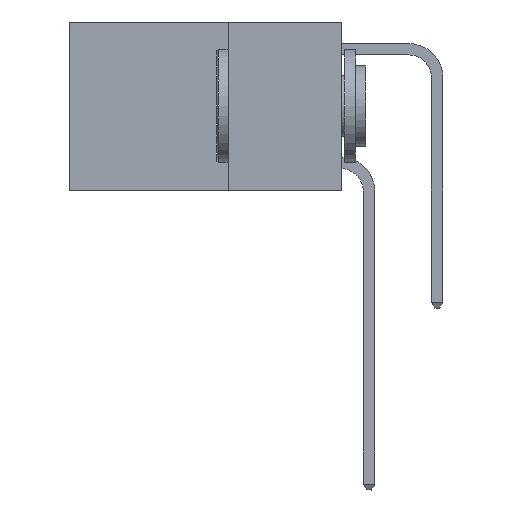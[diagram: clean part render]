
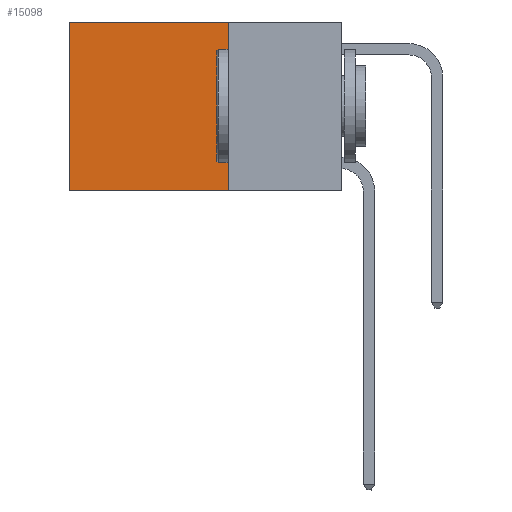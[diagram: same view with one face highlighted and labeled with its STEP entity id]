
A CAD part, left-side view. The second image highlights one B-rep face of the part: STEP entity #15098.
In plain terms, the highlighted planar face has unit normal (-1, 0, 0).
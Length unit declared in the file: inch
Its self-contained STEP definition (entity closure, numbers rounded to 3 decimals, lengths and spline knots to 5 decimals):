
#177 = VERTEX_POINT ( 'NONE', #13734 ) ;
#1425 = EDGE_LOOP ( 'NONE', ( #12288, #14603, #14387, #11942 ) ) ;
#2439 = LINE ( 'NONE', #4315, #9873 ) ;
#3101 = DIRECTION ( 'NONE',  ( 0., 0., -1. ) ) ;
#3390 = FACE_OUTER_BOUND ( 'NONE', #1425, .T. ) ;
#4002 = LINE ( 'NONE', #7908, #15254 ) ;
#4315 = CARTESIAN_POINT ( 'NONE',  ( 0.2625, 0.25, -0.37 ) ) ;
#5177 = DIRECTION ( 'NONE',  ( 0., 1., 0. ) ) ;
#5392 = CARTESIAN_POINT ( 'NONE',  ( 0.2625, 0.25, -0.37 ) ) ;
#5939 = VERTEX_POINT ( 'NONE', #7445 ) ;
#6036 = CARTESIAN_POINT ( 'NONE',  ( 0.2625, 0.25, 0. ) ) ;
#6421 = DIRECTION ( 'NONE',  ( 0., 0., -1. ) ) ;
#7288 = DIRECTION ( 'NONE',  ( 0., 1., 0. ) ) ;
#7445 = CARTESIAN_POINT ( 'NONE',  ( 0.2625, 0.6, 0. ) ) ;
#7856 = CARTESIAN_POINT ( 'NONE',  ( 0.2625, 0.6, -0.37 ) ) ;
#7908 = CARTESIAN_POINT ( 'NONE',  ( 0.2625, 0.25, 0. ) ) ;
#8926 = LINE ( 'NONE', #17455, #9383 ) ;
#9383 = VECTOR ( 'NONE', #18900, 39.37008 ) ;
#9873 = VECTOR ( 'NONE', #7288, 39.37008 ) ;
#10489 = VERTEX_POINT ( 'NONE', #7856 ) ;
#10540 = LINE ( 'NONE', #16834, #17766 ) ;
#11911 = DIRECTION ( 'NONE',  ( 1., 0., 0. ) ) ;
#11942 = ORIENTED_EDGE ( 'NONE', *, *, #15377, .T. ) ;
#12288 = ORIENTED_EDGE ( 'NONE', *, *, #15693, .T. ) ;
#12506 = VERTEX_POINT ( 'NONE', #5392 ) ;
#13734 = CARTESIAN_POINT ( 'NONE',  ( 0.2625, 0.25, 0. ) ) ;
#14009 = EDGE_CURVE ( 'NONE', #12506, #10489, #2439, .T. ) ;
#14387 = ORIENTED_EDGE ( 'NONE', *, *, #17076, .F. ) ;
#14603 = ORIENTED_EDGE ( 'NONE', *, *, #14009, .F. ) ;
#15093 = AXIS2_PLACEMENT_3D ( 'NONE', #6036, #11911, #3101 ) ;
#15098 = ADVANCED_FACE ( 'NONE', ( #3390 ), #17658, .F. ) ;
#15254 = VECTOR ( 'NONE', #6421, 39.37008 ) ;
#15377 = EDGE_CURVE ( 'NONE', #177, #5939, #10540, .T. ) ;
#15693 = EDGE_CURVE ( 'NONE', #5939, #10489, #8926, .T. ) ;
#16834 = CARTESIAN_POINT ( 'NONE',  ( 0.2625, 0.25, 0. ) ) ;
#17076 = EDGE_CURVE ( 'NONE', #177, #12506, #4002, .T. ) ;
#17455 = CARTESIAN_POINT ( 'NONE',  ( 0.2625, 0.6, 0. ) ) ;
#17658 = PLANE ( 'NONE',  #15093 ) ;
#17766 = VECTOR ( 'NONE', #5177, 39.37008 ) ;
#18900 = DIRECTION ( 'NONE',  ( 0., 0., -1. ) ) ;
